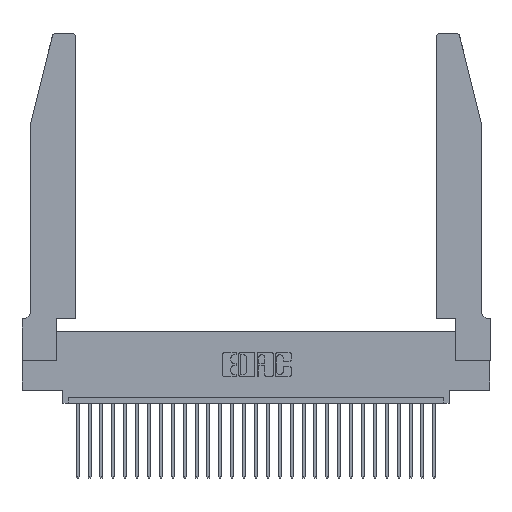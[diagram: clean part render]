
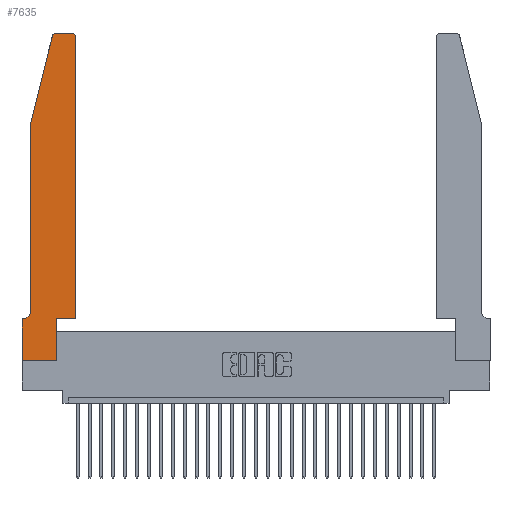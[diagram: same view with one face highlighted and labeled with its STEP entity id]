
A CAD part, top view. The second image highlights one B-rep face of the part: STEP entity #7635.
In plain terms, the highlighted planar face has unit normal (0, 0, 1).
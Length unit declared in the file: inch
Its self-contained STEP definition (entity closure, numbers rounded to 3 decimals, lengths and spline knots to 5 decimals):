
#242 = VECTOR ( 'NONE', #16937, 39.37008 ) ;
#294 = CARTESIAN_POINT ( 'NONE',  ( 0.4505, 0.35, 0.37 ) ) ;
#327 = CARTESIAN_POINT ( 'NONE',  ( 0., 0.35, 0.37 ) ) ;
#1156 = CARTESIAN_POINT ( 'NONE',  ( 0.2865, 0., 0.37 ) ) ;
#1251 = DIRECTION ( 'NONE',  ( 1., 0., 0. ) ) ;
#1615 = CARTESIAN_POINT ( 'NONE',  ( 0.0755, 2., 0.37 ) ) ;
#2015 = AXIS2_PLACEMENT_3D ( 'NONE', #327, #7653, #25956 ) ;
#2088 = VECTOR ( 'NONE', #5068, 39.37008 ) ;
#2229 = CARTESIAN_POINT ( 'NONE',  ( 0., 0., 0.37 ) ) ;
#2306 = DIRECTION ( 'NONE',  ( 0., 1., 0. ) ) ;
#2324 = LINE ( 'NONE', #294, #27041 ) ;
#2529 = EDGE_CURVE ( 'NONE', #7762, #21780, #7634, .T. ) ;
#2618 = EDGE_CURVE ( 'NONE', #27986, #8295, #12634, .T. ) ;
#2639 = CARTESIAN_POINT ( 'NONE',  ( 0.4505, 0.35, 0.37 ) ) ;
#2703 = AXIS2_PLACEMENT_3D ( 'NONE', #9494, #18318, #16130 ) ;
#3272 = DIRECTION ( 'NONE',  ( 1., 0., 0. ) ) ;
#3426 = ORIENTED_EDGE ( 'NONE', *, *, #16516, .T. ) ;
#3856 = CARTESIAN_POINT ( 'NONE',  ( 0.284, 2.72, 0.37 ) ) ;
#3978 = VECTOR ( 'NONE', #28604, 39.37008 ) ;
#3979 = CARTESIAN_POINT ( 'NONE',  ( 0.4505, 0.35, 0.37 ) ) ;
#4611 = CARTESIAN_POINT ( 'NONE',  ( 0.0055, 0.35, 0.37 ) ) ;
#5068 = DIRECTION ( 'NONE',  ( 0., -1., 0. ) ) ;
#5070 = EDGE_CURVE ( 'NONE', #10954, #27026, #7122, .T. ) ;
#6529 = CARTESIAN_POINT ( 'NONE',  ( 0.4205, 2.75, 0.37 ) ) ;
#7122 = CIRCLE ( 'NONE', #23699, 0.03 ) ;
#7377 = VERTEX_POINT ( 'NONE', #1156 ) ;
#7388 = VERTEX_POINT ( 'NONE', #28620 ) ;
#7634 = LINE ( 'NONE', #18228, #24472 ) ;
#7635 = ADVANCED_FACE ( 'NONE', ( #26586 ), #27793, .T. ) ;
#7653 = DIRECTION ( 'NONE',  ( 0., 0., 1. ) ) ;
#7762 = VERTEX_POINT ( 'NONE', #16409 ) ;
#8156 = CARTESIAN_POINT ( 'NONE',  ( 0.0755, 0.35, 0.37 ) ) ;
#8295 = VERTEX_POINT ( 'NONE', #4611 ) ;
#8474 = ORIENTED_EDGE ( 'NONE', *, *, #17469, .T. ) ;
#8514 = AXIS2_PLACEMENT_3D ( 'NONE', #23794, #19665, #1251 ) ;
#9244 = ORIENTED_EDGE ( 'NONE', *, *, #27211, .T. ) ;
#9494 = CARTESIAN_POINT ( 'NONE',  ( 0.0055, 0.42, 0.37 ) ) ;
#9520 = CIRCLE ( 'NONE', #8514, 0.03 ) ;
#9793 = LINE ( 'NONE', #27018, #24884 ) ;
#10191 = CARTESIAN_POINT ( 'NONE',  ( 0.284, 2.75, 0.37 ) ) ;
#10954 = VERTEX_POINT ( 'NONE', #10191 ) ;
#11053 = ORIENTED_EDGE ( 'NONE', *, *, #2618, .T. ) ;
#12634 = CIRCLE ( 'NONE', #2703, 0.07 ) ;
#13049 = EDGE_CURVE ( 'NONE', #21054, #18331, #27949, .T. ) ;
#14427 = ORIENTED_EDGE ( 'NONE', *, *, #27603, .T. ) ;
#14643 = CARTESIAN_POINT ( 'NONE',  ( 0., 0., 0.37 ) ) ;
#14706 = ORIENTED_EDGE ( 'NONE', *, *, #2529, .T. ) ;
#15133 = EDGE_CURVE ( 'NONE', #7388, #27986, #17131, .T. ) ;
#15444 = ORIENTED_EDGE ( 'NONE', *, *, #5070, .T. ) ;
#15596 = ORIENTED_EDGE ( 'NONE', *, *, #15133, .T. ) ;
#16130 = DIRECTION ( 'NONE',  ( -1., 0., 0. ) ) ;
#16166 = CARTESIAN_POINT ( 'NONE',  ( 0.2865, 0.35, 0.37 ) ) ;
#16281 = CARTESIAN_POINT ( 'NONE',  ( 0.2865, 0.35, 0.37 ) ) ;
#16409 = CARTESIAN_POINT ( 'NONE',  ( 0., 0.35, 0.37 ) ) ;
#16487 = LINE ( 'NONE', #8156, #3978 ) ;
#16516 = EDGE_CURVE ( 'NONE', #19124, #27002, #9520, .T. ) ;
#16937 = DIRECTION ( 'NONE',  ( 1., 0., 0. ) ) ;
#17131 = LINE ( 'NONE', #29717, #2088 ) ;
#17469 = EDGE_CURVE ( 'NONE', #7377, #21054, #18068, .T. ) ;
#17622 = DIRECTION ( 'NONE',  ( -0.239, -0.971, 0. ) ) ;
#17979 = DIRECTION ( 'NONE',  ( 0., 1., 0. ) ) ;
#18068 = LINE ( 'NONE', #16166, #18434 ) ;
#18228 = CARTESIAN_POINT ( 'NONE',  ( 0., 0., 0.37 ) ) ;
#18318 = DIRECTION ( 'NONE',  ( 0., 0., -1. ) ) ;
#18331 = VERTEX_POINT ( 'NONE', #3979 ) ;
#18434 = VECTOR ( 'NONE', #17979, 39.37008 ) ;
#18459 = DIRECTION ( 'NONE',  ( 1., 0., 0. ) ) ;
#19036 = VECTOR ( 'NONE', #17622, 39.37008 ) ;
#19124 = VERTEX_POINT ( 'NONE', #27946 ) ;
#19665 = DIRECTION ( 'NONE',  ( 0., 0., 1. ) ) ;
#20015 = EDGE_CURVE ( 'NONE', #27026, #7388, #27629, .T. ) ;
#21054 = VERTEX_POINT ( 'NONE', #16281 ) ;
#21212 = EDGE_CURVE ( 'NONE', #8295, #7762, #16487, .T. ) ;
#21780 = VERTEX_POINT ( 'NONE', #2229 ) ;
#21960 = ORIENTED_EDGE ( 'NONE', *, *, #21212, .T. ) ;
#22155 = DIRECTION ( 'NONE',  ( 0., 0., 1. ) ) ;
#22309 = VECTOR ( 'NONE', #3272, 39.37008 ) ;
#22386 = ORIENTED_EDGE ( 'NONE', *, *, #20015, .T. ) ;
#22568 = DIRECTION ( 'NONE',  ( 0., -1., 0. ) ) ;
#23699 = AXIS2_PLACEMENT_3D ( 'NONE', #3856, #22155, #18459 ) ;
#23794 = CARTESIAN_POINT ( 'NONE',  ( 0.4205, 2.72, 0.37 ) ) ;
#24472 = VECTOR ( 'NONE', #22568, 39.37008 ) ;
#24884 = VECTOR ( 'NONE', #29352, 39.37008 ) ;
#25379 = EDGE_CURVE ( 'NONE', #21780, #7377, #27699, .T. ) ;
#25956 = DIRECTION ( 'NONE',  ( 1., 0., 0. ) ) ;
#26586 = FACE_OUTER_BOUND ( 'NONE', #27179, .T. ) ;
#27002 = VERTEX_POINT ( 'NONE', #6529 ) ;
#27018 = CARTESIAN_POINT ( 'NONE',  ( 0.2605, 2.75, 0.37 ) ) ;
#27026 = VERTEX_POINT ( 'NONE', #29484 ) ;
#27041 = VECTOR ( 'NONE', #2306, 39.37008 ) ;
#27179 = EDGE_LOOP ( 'NONE', ( #14427, #15444, #22386, #15596, #11053, #21960, #14706, #29004, #8474, #28685, #9244, #3426 ) ) ;
#27211 = EDGE_CURVE ( 'NONE', #18331, #19124, #2324, .T. ) ;
#27603 = EDGE_CURVE ( 'NONE', #27002, #10954, #9793, .T. ) ;
#27629 = LINE ( 'NONE', #1615, #19036 ) ;
#27699 = LINE ( 'NONE', #14643, #22309 ) ;
#27793 = PLANE ( 'NONE',  #2015 ) ;
#27946 = CARTESIAN_POINT ( 'NONE',  ( 0.4505, 2.72, 0.37 ) ) ;
#27949 = LINE ( 'NONE', #2639, #242 ) ;
#27986 = VERTEX_POINT ( 'NONE', #28739 ) ;
#28604 = DIRECTION ( 'NONE',  ( -1., 0., 0. ) ) ;
#28620 = CARTESIAN_POINT ( 'NONE',  ( 0.0755, 2., 0.37 ) ) ;
#28685 = ORIENTED_EDGE ( 'NONE', *, *, #13049, .T. ) ;
#28739 = CARTESIAN_POINT ( 'NONE',  ( 0.0755, 0.42, 0.37 ) ) ;
#29004 = ORIENTED_EDGE ( 'NONE', *, *, #25379, .T. ) ;
#29352 = DIRECTION ( 'NONE',  ( -1., 0., 0. ) ) ;
#29484 = CARTESIAN_POINT ( 'NONE',  ( 0.25487, 2.72718, 0.37 ) ) ;
#29717 = CARTESIAN_POINT ( 'NONE',  ( 0.0755, 2., 0.37 ) ) ;
